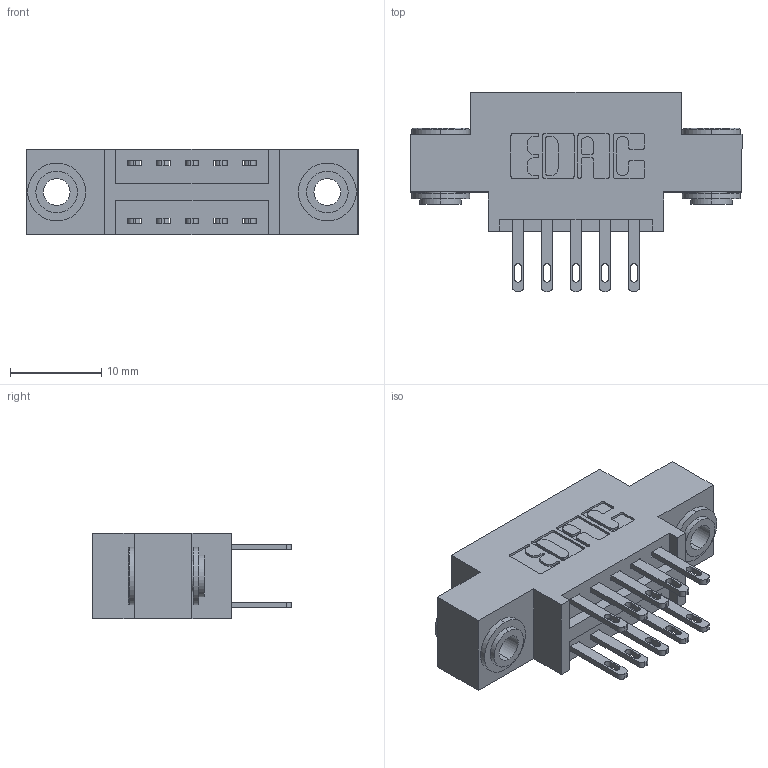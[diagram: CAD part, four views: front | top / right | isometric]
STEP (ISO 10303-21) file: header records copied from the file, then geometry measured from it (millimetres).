
FILE_DESCRIPTION (( 'STEP AP203' ), '1' );
FILE_NAME ('346-010-500-803.STEP', '2022-05-17T16:26:34', ( '' ), ( '' ), 'SwSTEP 2.0', 'SolidWorks 2020', '' );
FILE_SCHEMA (( 'CONFIG_CONTROL_DESIGN' ));
Length unit declared in the file: inch
Products named in the file (4): 345-250-002_345-250-002-102; 345-292-001_345-293-100; 346-010-500-803; 346 Part_0.170 Offset - 0.156 Dia-TH
Assembly tree (13 placements, depth 2):
  346-010-500-803
    346 Part_0.170 Offset - 0.156 Dia-TH
    345-292-001_345-293-100  x10
    345-250-002_345-250-002-102  x2
Bounding box: 36.45 x 21.84 x 9.4 mm (x, y, z)
Volume: 3144.1 mm3; surface area: 4273.2 mm2
Topology: 13 solids, 13 shells, 658 faces, 1923 edges, 1278 vertices
Faces by surface type: plane 394, cylinder 256, cone 8
Entity records: 9372 total; most frequent: CARTESIAN_POINT 1577, ORIENTED_EDGE 1502, DIRECTION 1473, EDGE_CURVE 751, LINE 571, VECTOR 571, VERTEX_POINT 498, AXIS2_PLACEMENT_3D 451
